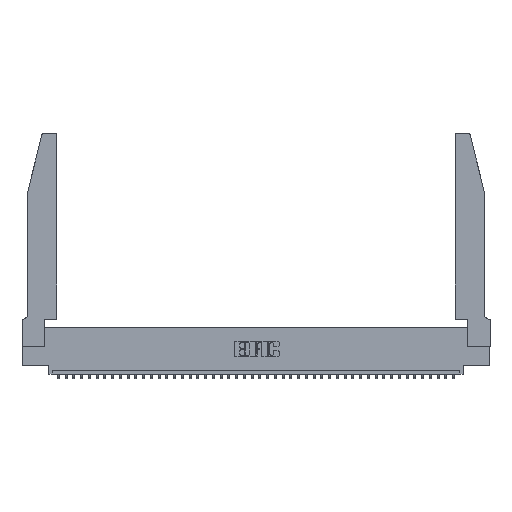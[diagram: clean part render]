
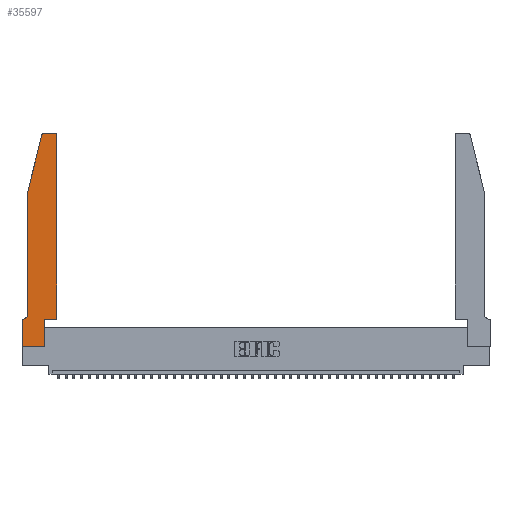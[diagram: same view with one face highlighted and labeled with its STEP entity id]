
A CAD part, top view. The second image highlights one B-rep face of the part: STEP entity #35597.
In plain terms, the highlighted planar face has unit normal (0, 0, 1).
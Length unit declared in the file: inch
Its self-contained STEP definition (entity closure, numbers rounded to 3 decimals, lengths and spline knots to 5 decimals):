
#152 = DIRECTION ( 'NONE',  ( 0., 0., -1. ) ) ;
#1121 = EDGE_CURVE ( 'NONE', #22881, #33343, #10560, .T. ) ;
#1149 = EDGE_CURVE ( 'NONE', #25883, #8865, #13139, .T. ) ;
#2061 = DIRECTION ( 'NONE',  ( 1., 0., 0. ) ) ;
#2802 = VERTEX_POINT ( 'NONE', #16599 ) ;
#3626 = CARTESIAN_POINT ( 'NONE',  ( 0.0755, 2., 0.37 ) ) ;
#3694 = EDGE_CURVE ( 'NONE', #10801, #22881, #36521, .T. ) ;
#3870 = VECTOR ( 'NONE', #10254, 39.37008 ) ;
#4066 = VECTOR ( 'NONE', #25317, 39.37008 ) ;
#4455 = DIRECTION ( 'NONE',  ( 0., -1., 0. ) ) ;
#4466 = VERTEX_POINT ( 'NONE', #37940 ) ;
#4930 = VERTEX_POINT ( 'NONE', #17225 ) ;
#4936 = VECTOR ( 'NONE', #4455, 39.37008 ) ;
#5294 = DIRECTION ( 'NONE',  ( 0., 1., 0. ) ) ;
#5885 = VECTOR ( 'NONE', #5294, 39.37008 ) ;
#8865 = VERTEX_POINT ( 'NONE', #32431 ) ;
#9079 = AXIS2_PLACEMENT_3D ( 'NONE', #9778, #32647, #32791 ) ;
#9778 = CARTESIAN_POINT ( 'NONE',  ( 0., 0.35, 0.37 ) ) ;
#10254 = DIRECTION ( 'NONE',  ( 0., -1., 0. ) ) ;
#10560 = CIRCLE ( 'NONE', #42172, 0.03 ) ;
#10801 = VERTEX_POINT ( 'NONE', #40801 ) ;
#11781 = LINE ( 'NONE', #23755, #42779 ) ;
#11970 = CARTESIAN_POINT ( 'NONE',  ( 0., 0.35, 0.37 ) ) ;
#13139 = CIRCLE ( 'NONE', #21448, 0.07 ) ;
#13421 = DIRECTION ( 'NONE',  ( 0., 0., 1. ) ) ;
#13458 = ORIENTED_EDGE ( 'NONE', *, *, #35050, .T. ) ;
#13975 = CARTESIAN_POINT ( 'NONE',  ( 0.284, 2.75, 0.37 ) ) ;
#14239 = ORIENTED_EDGE ( 'NONE', *, *, #1149, .T. ) ;
#14337 = DIRECTION ( 'NONE',  ( -1., 0., 0. ) ) ;
#15130 = LINE ( 'NONE', #18884, #5885 ) ;
#15140 = DIRECTION ( 'NONE',  ( -0.239, -0.971, 0. ) ) ;
#15216 = LINE ( 'NONE', #3626, #3870 ) ;
#15380 = VERTEX_POINT ( 'NONE', #11970 ) ;
#15777 = EDGE_CURVE ( 'NONE', #27944, #4930, #32529, .T. ) ;
#16175 = FACE_OUTER_BOUND ( 'NONE', #24513, .T. ) ;
#16599 = CARTESIAN_POINT ( 'NONE',  ( 0., 0., 0.37 ) ) ;
#16955 = LINE ( 'NONE', #34584, #27244 ) ;
#17098 = EDGE_CURVE ( 'NONE', #31216, #27944, #15130, .T. ) ;
#17225 = CARTESIAN_POINT ( 'NONE',  ( 0.4505, 0.35, 0.37 ) ) ;
#17790 = ORIENTED_EDGE ( 'NONE', *, *, #15777, .T. ) ;
#18034 = CARTESIAN_POINT ( 'NONE',  ( 0., 0., 0.37 ) ) ;
#18884 = CARTESIAN_POINT ( 'NONE',  ( 0.2865, 0.35, 0.37 ) ) ;
#19391 = LINE ( 'NONE', #27795, #34776 ) ;
#19446 = CARTESIAN_POINT ( 'NONE',  ( 0.0755, 0.42, 0.37 ) ) ;
#19482 = EDGE_CURVE ( 'NONE', #2802, #31216, #16955, .T. ) ;
#19485 = ORIENTED_EDGE ( 'NONE', *, *, #24805, .T. ) ;
#21448 = AXIS2_PLACEMENT_3D ( 'NONE', #29804, #152, #30344 ) ;
#21567 = CARTESIAN_POINT ( 'NONE',  ( 0.4505, 0.35, 0.37 ) ) ;
#22302 = ORIENTED_EDGE ( 'NONE', *, *, #40927, .T. ) ;
#22784 = ORIENTED_EDGE ( 'NONE', *, *, #38553, .T. ) ;
#22881 = VERTEX_POINT ( 'NONE', #13975 ) ;
#22915 = DIRECTION ( 'NONE',  ( 0., 0., 1. ) ) ;
#23449 = CIRCLE ( 'NONE', #37048, 0.03 ) ;
#23755 = CARTESIAN_POINT ( 'NONE',  ( 0.0755, 0.35, 0.37 ) ) ;
#23802 = CARTESIAN_POINT ( 'NONE',  ( 0.284, 2.72, 0.37 ) ) ;
#24513 = EDGE_LOOP ( 'NONE', ( #37049, #26732, #22302, #13458, #14239, #22784, #19485, #35722, #31592, #17790, #26089, #41697 ) ) ;
#24722 = CARTESIAN_POINT ( 'NONE',  ( 0.2865, 0.35, 0.37 ) ) ;
#24805 = EDGE_CURVE ( 'NONE', #15380, #2802, #35851, .T. ) ;
#25317 = DIRECTION ( 'NONE',  ( -1., 0., 0. ) ) ;
#25883 = VERTEX_POINT ( 'NONE', #19446 ) ;
#26089 = ORIENTED_EDGE ( 'NONE', *, *, #35126, .T. ) ;
#26525 = DIRECTION ( 'NONE',  ( 1., 0., 0. ) ) ;
#26732 = ORIENTED_EDGE ( 'NONE', *, *, #1121, .T. ) ;
#27244 = VECTOR ( 'NONE', #2061, 39.37008 ) ;
#27668 = CARTESIAN_POINT ( 'NONE',  ( 0.0755, 2., 0.37 ) ) ;
#27795 = CARTESIAN_POINT ( 'NONE',  ( 0.4505, 0.35, 0.37 ) ) ;
#27944 = VERTEX_POINT ( 'NONE', #24722 ) ;
#28486 = CARTESIAN_POINT ( 'NONE',  ( 0.2865, 0., 0.37 ) ) ;
#28633 = VECTOR ( 'NONE', #15140, 39.37008 ) ;
#29463 = DIRECTION ( 'NONE',  ( 1., 0., 0. ) ) ;
#29804 = CARTESIAN_POINT ( 'NONE',  ( 0.0055, 0.42, 0.37 ) ) ;
#30344 = DIRECTION ( 'NONE',  ( -1., 0., 0. ) ) ;
#30776 = DIRECTION ( 'NONE',  ( 0., 1., 0. ) ) ;
#31216 = VERTEX_POINT ( 'NONE', #28486 ) ;
#31592 = ORIENTED_EDGE ( 'NONE', *, *, #17098, .T. ) ;
#32361 = CARTESIAN_POINT ( 'NONE',  ( 0.25487, 2.72718, 0.37 ) ) ;
#32431 = CARTESIAN_POINT ( 'NONE',  ( 0.0055, 0.35, 0.37 ) ) ;
#32529 = LINE ( 'NONE', #21567, #42397 ) ;
#32647 = DIRECTION ( 'NONE',  ( 0., 0., 1. ) ) ;
#32791 = DIRECTION ( 'NONE',  ( 1., 0., 0. ) ) ;
#33076 = PLANE ( 'NONE',  #9079 ) ;
#33343 = VERTEX_POINT ( 'NONE', #32361 ) ;
#34584 = CARTESIAN_POINT ( 'NONE',  ( 0., 0., 0.37 ) ) ;
#34776 = VECTOR ( 'NONE', #30776, 39.37008 ) ;
#35050 = EDGE_CURVE ( 'NONE', #35206, #25883, #15216, .T. ) ;
#35126 = EDGE_CURVE ( 'NONE', #4930, #4466, #19391, .T. ) ;
#35206 = VERTEX_POINT ( 'NONE', #41707 ) ;
#35484 = CARTESIAN_POINT ( 'NONE',  ( 0.2605, 2.75, 0.37 ) ) ;
#35597 = ADVANCED_FACE ( 'NONE', ( #16175 ), #33076, .T. ) ;
#35722 = ORIENTED_EDGE ( 'NONE', *, *, #19482, .T. ) ;
#35851 = LINE ( 'NONE', #18034, #4936 ) ;
#36112 = CARTESIAN_POINT ( 'NONE',  ( 0.4205, 2.72, 0.37 ) ) ;
#36521 = LINE ( 'NONE', #35484, #4066 ) ;
#37048 = AXIS2_PLACEMENT_3D ( 'NONE', #36112, #22915, #29463 ) ;
#37049 = ORIENTED_EDGE ( 'NONE', *, *, #3694, .T. ) ;
#37940 = CARTESIAN_POINT ( 'NONE',  ( 0.4505, 2.72, 0.37 ) ) ;
#38553 = EDGE_CURVE ( 'NONE', #8865, #15380, #11781, .T. ) ;
#40801 = CARTESIAN_POINT ( 'NONE',  ( 0.4205, 2.75, 0.37 ) ) ;
#40927 = EDGE_CURVE ( 'NONE', #33343, #35206, #42129, .T. ) ;
#41451 = DIRECTION ( 'NONE',  ( 1., 0., 0. ) ) ;
#41697 = ORIENTED_EDGE ( 'NONE', *, *, #41728, .T. ) ;
#41707 = CARTESIAN_POINT ( 'NONE',  ( 0.0755, 2., 0.37 ) ) ;
#41728 = EDGE_CURVE ( 'NONE', #4466, #10801, #23449, .T. ) ;
#42129 = LINE ( 'NONE', #27668, #28633 ) ;
#42172 = AXIS2_PLACEMENT_3D ( 'NONE', #23802, #13421, #26525 ) ;
#42397 = VECTOR ( 'NONE', #41451, 39.37008 ) ;
#42779 = VECTOR ( 'NONE', #14337, 39.37008 ) ;
